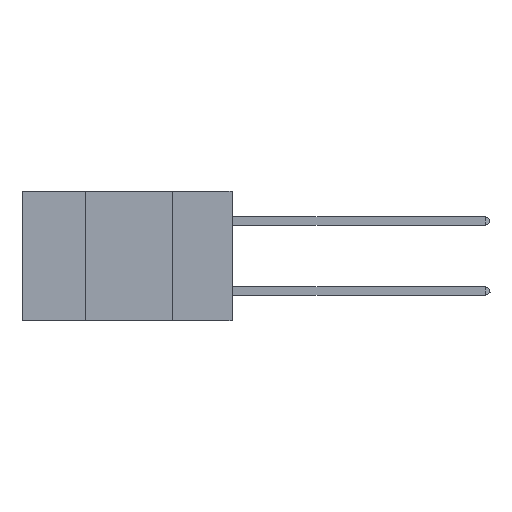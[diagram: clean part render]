
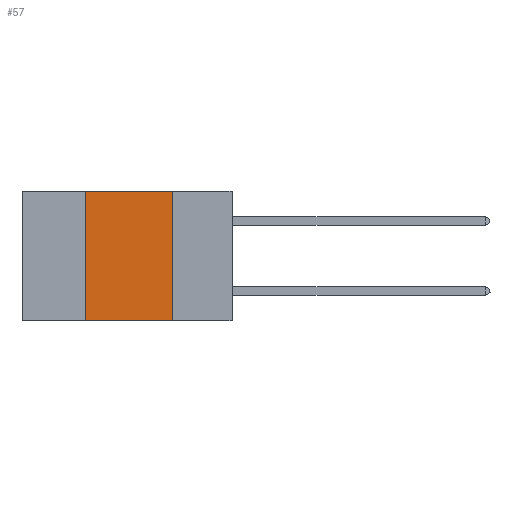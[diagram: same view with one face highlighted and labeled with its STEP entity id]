
A CAD part, left-side view. The second image highlights one B-rep face of the part: STEP entity #57.
In plain terms, the highlighted planar face has unit normal (-1, 0, 0).
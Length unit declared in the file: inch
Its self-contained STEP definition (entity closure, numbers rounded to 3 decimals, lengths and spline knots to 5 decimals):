
#57 = ADVANCED_FACE ( 'NONE', ( #8975 ), #13923, .F. ) ;
#488 = VERTEX_POINT ( 'NONE', #12282 ) ;
#849 = CARTESIAN_POINT ( 'NONE',  ( 0., 0.6, 0. ) ) ;
#1211 = LINE ( 'NONE', #10700, #9909 ) ;
#1611 = EDGE_LOOP ( 'NONE', ( #8052, #6930, #10911, #13300 ) ) ;
#2268 = DIRECTION ( 'NONE',  ( 1., 0., 0. ) ) ;
#2368 = DIRECTION ( 'NONE',  ( 0., 0., 1. ) ) ;
#2425 = CARTESIAN_POINT ( 'NONE',  ( 0., 0.42, 0. ) ) ;
#2602 = EDGE_CURVE ( 'NONE', #11588, #8675, #5296, .T. ) ;
#3040 = EDGE_CURVE ( 'NONE', #11588, #4228, #9057, .T. ) ;
#3610 = AXIS2_PLACEMENT_3D ( 'NONE', #14233, #2268, #4764 ) ;
#3656 = CARTESIAN_POINT ( 'NONE',  ( 0., 0.42, 0. ) ) ;
#4228 = VERTEX_POINT ( 'NONE', #5749 ) ;
#4764 = DIRECTION ( 'NONE',  ( 0., 0., -1. ) ) ;
#5296 = LINE ( 'NONE', #2425, #15255 ) ;
#5615 = VECTOR ( 'NONE', #10512, 39.37008 ) ;
#5683 = CARTESIAN_POINT ( 'NONE',  ( 0., 0.6, -0.37 ) ) ;
#5749 = CARTESIAN_POINT ( 'NONE',  ( 0., 0.17, -0.37 ) ) ;
#6209 = VECTOR ( 'NONE', #10410, 39.37008 ) ;
#6581 = EDGE_CURVE ( 'NONE', #488, #4228, #1211, .T. ) ;
#6930 = ORIENTED_EDGE ( 'NONE', *, *, #10293, .F. ) ;
#8052 = ORIENTED_EDGE ( 'NONE', *, *, #6581, .F. ) ;
#8675 = VERTEX_POINT ( 'NONE', #3656 ) ;
#8975 = FACE_OUTER_BOUND ( 'NONE', #1611, .T. ) ;
#9057 = LINE ( 'NONE', #5683, #6209 ) ;
#9909 = VECTOR ( 'NONE', #10067, 39.37008 ) ;
#10067 = DIRECTION ( 'NONE',  ( 0., 0., -1. ) ) ;
#10234 = CARTESIAN_POINT ( 'NONE',  ( 0., 0.42, -0.37 ) ) ;
#10293 = EDGE_CURVE ( 'NONE', #8675, #488, #12961, .T. ) ;
#10410 = DIRECTION ( 'NONE',  ( 0., -1., 0. ) ) ;
#10512 = DIRECTION ( 'NONE',  ( 0., -1., 0. ) ) ;
#10700 = CARTESIAN_POINT ( 'NONE',  ( 0., 0.17, 0. ) ) ;
#10911 = ORIENTED_EDGE ( 'NONE', *, *, #2602, .F. ) ;
#11588 = VERTEX_POINT ( 'NONE', #10234 ) ;
#12282 = CARTESIAN_POINT ( 'NONE',  ( 0., 0.17, 0. ) ) ;
#12961 = LINE ( 'NONE', #849, #5615 ) ;
#13300 = ORIENTED_EDGE ( 'NONE', *, *, #3040, .T. ) ;
#13923 = PLANE ( 'NONE',  #3610 ) ;
#14233 = CARTESIAN_POINT ( 'NONE',  ( 0., 0.6, 0. ) ) ;
#15255 = VECTOR ( 'NONE', #2368, 39.37008 ) ;
